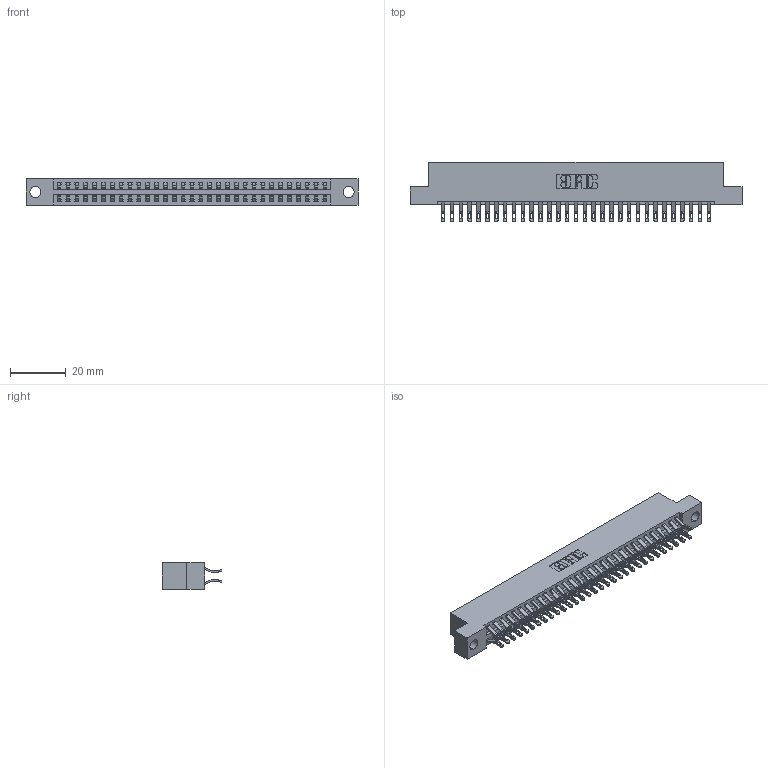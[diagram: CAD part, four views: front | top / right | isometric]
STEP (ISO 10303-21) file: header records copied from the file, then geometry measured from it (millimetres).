
FILE_DESCRIPTION (( 'STEP AP203' ), '1' );
FILE_NAME ('346-062-555-204.STEP', '2022-05-24T14:01:44', ( '' ), ( '' ), 'SwSTEP 2.0', 'SolidWorks 2020', '' );
FILE_SCHEMA (( 'CONFIG_CONTROL_DESIGN' ));
Length unit declared in the file: inch
Products named in the file (3): 345-292-001_555 Tail; 346 Part_Flush Mounting Lugs - 0.156 Dia-TH; 346-062-555-204
Assembly tree (63 placements, depth 2):
  346-062-555-204
    346 Part_Flush Mounting Lugs - 0.156 Dia-TH
    345-292-001_555 Tail  x62
Bounding box: 119 x 21.46 x 9.4 mm (x, y, z)
Volume: 11592.3 mm3; surface area: 16250.5 mm2
Topology: 63 solids, 63 shells, 3732 faces, 11711 edges, 7806 vertices
Faces by surface type: plane 2136, cylinder 1596
Entity records: 22457 total; most frequent: CARTESIAN_POINT 3756, ORIENTED_EDGE 3658, DIRECTION 3329, EDGE_CURVE 1829, LINE 1553, VECTOR 1553, VERTEX_POINT 1218, AXIS2_PLACEMENT_3D 888
